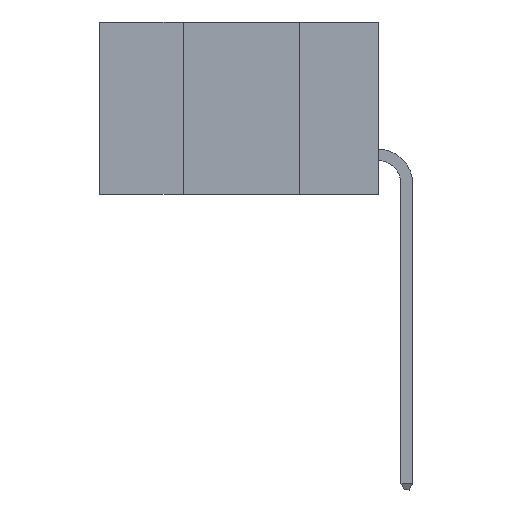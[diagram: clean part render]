
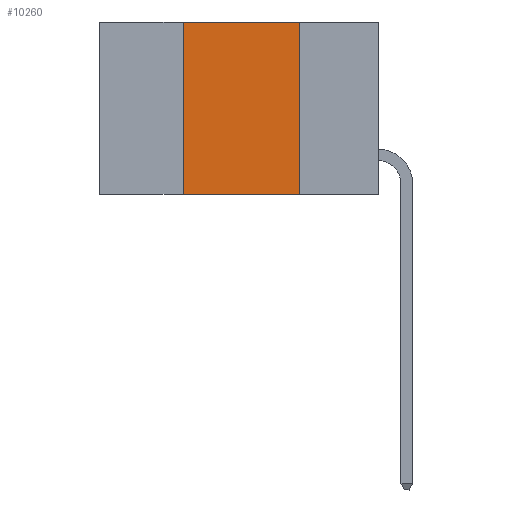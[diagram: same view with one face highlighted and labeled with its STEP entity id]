
A CAD part, left-side view. The second image highlights one B-rep face of the part: STEP entity #10260.
In plain terms, the highlighted planar face has unit normal (-1, 0, 0).
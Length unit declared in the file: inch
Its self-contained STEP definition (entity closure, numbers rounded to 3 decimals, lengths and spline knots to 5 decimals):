
#377 = LINE ( 'NONE', #11554, #7488 ) ;
#557 = LINE ( 'NONE', #1273, #3813 ) ;
#673 = VERTEX_POINT ( 'NONE', #10395 ) ;
#687 = CARTESIAN_POINT ( 'NONE',  ( 0., 0.42, -0.37 ) ) ;
#859 = DIRECTION ( 'NONE',  ( 0., 0., -1. ) ) ;
#873 = ORIENTED_EDGE ( 'NONE', *, *, #7430, .T. ) ;
#1057 = VERTEX_POINT ( 'NONE', #10173 ) ;
#1244 = ORIENTED_EDGE ( 'NONE', *, *, #5946, .F. ) ;
#1273 = CARTESIAN_POINT ( 'NONE',  ( 0., 0.42, 0. ) ) ;
#1399 = EDGE_LOOP ( 'NONE', ( #11278, #5625, #1244, #873 ) ) ;
#1791 = CARTESIAN_POINT ( 'NONE',  ( 0., 0.6, 0. ) ) ;
#2247 = CARTESIAN_POINT ( 'NONE',  ( 0., 0.17, -0.37 ) ) ;
#2380 = LINE ( 'NONE', #6887, #7244 ) ;
#3262 = DIRECTION ( 'NONE',  ( 0., 0., -1. ) ) ;
#3369 = VERTEX_POINT ( 'NONE', #2247 ) ;
#3813 = VECTOR ( 'NONE', #10447, 39.37008 ) ;
#4422 = CARTESIAN_POINT ( 'NONE',  ( 0., 0.6, 0. ) ) ;
#5391 = EDGE_CURVE ( 'NONE', #673, #3369, #2380, .T. ) ;
#5576 = AXIS2_PLACEMENT_3D ( 'NONE', #1791, #10073, #859 ) ;
#5625 = ORIENTED_EDGE ( 'NONE', *, *, #6409, .F. ) ;
#5858 = DIRECTION ( 'NONE',  ( 0., -1., 0. ) ) ;
#5946 = EDGE_CURVE ( 'NONE', #7991, #1057, #557, .T. ) ;
#6409 = EDGE_CURVE ( 'NONE', #1057, #673, #11591, .T. ) ;
#6441 = PLANE ( 'NONE',  #5576 ) ;
#6887 = CARTESIAN_POINT ( 'NONE',  ( 0., 0.17, 0. ) ) ;
#7244 = VECTOR ( 'NONE', #3262, 39.37008 ) ;
#7430 = EDGE_CURVE ( 'NONE', #7991, #3369, #377, .T. ) ;
#7488 = VECTOR ( 'NONE', #5858, 39.37008 ) ;
#7991 = VERTEX_POINT ( 'NONE', #687 ) ;
#8270 = FACE_OUTER_BOUND ( 'NONE', #1399, .T. ) ;
#8987 = DIRECTION ( 'NONE',  ( 0., -1., 0. ) ) ;
#10073 = DIRECTION ( 'NONE',  ( 1., 0., 0. ) ) ;
#10173 = CARTESIAN_POINT ( 'NONE',  ( 0., 0.42, 0. ) ) ;
#10260 = ADVANCED_FACE ( 'NONE', ( #8270 ), #6441, .F. ) ;
#10395 = CARTESIAN_POINT ( 'NONE',  ( 0., 0.17, 0. ) ) ;
#10447 = DIRECTION ( 'NONE',  ( 0., 0., 1. ) ) ;
#10751 = VECTOR ( 'NONE', #8987, 39.37008 ) ;
#11278 = ORIENTED_EDGE ( 'NONE', *, *, #5391, .F. ) ;
#11554 = CARTESIAN_POINT ( 'NONE',  ( 0., 0.6, -0.37 ) ) ;
#11591 = LINE ( 'NONE', #4422, #10751 ) ;
